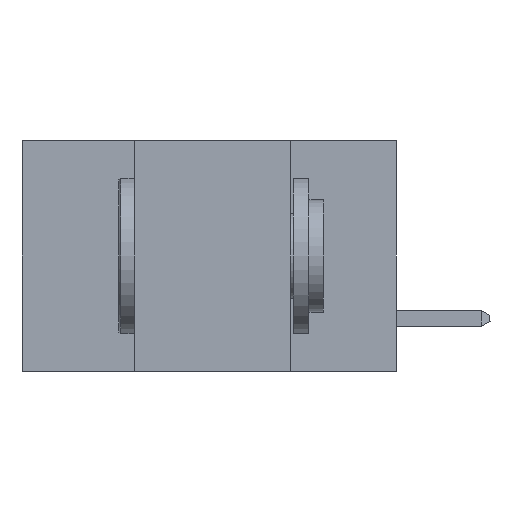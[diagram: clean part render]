
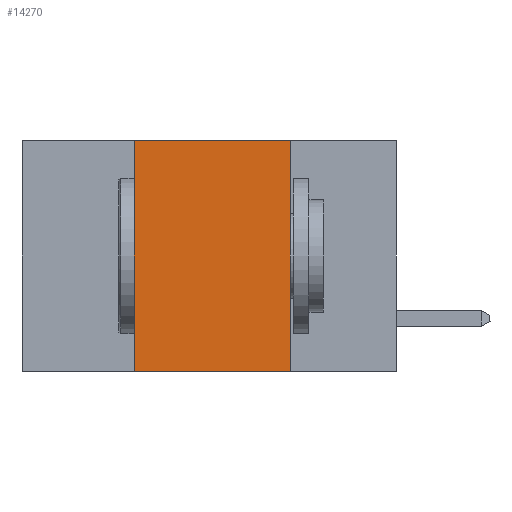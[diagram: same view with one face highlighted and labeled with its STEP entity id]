
A CAD part, left-side view. The second image highlights one B-rep face of the part: STEP entity #14270.
In plain terms, the highlighted planar face has unit normal (-1, 0, 0).
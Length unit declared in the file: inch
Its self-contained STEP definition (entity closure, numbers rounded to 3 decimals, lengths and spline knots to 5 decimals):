
#33 = DIRECTION ( 'NONE',  ( 0., 0., 1. ) ) ;
#756 = ORIENTED_EDGE ( 'NONE', *, *, #10860, .F. ) ;
#1103 = LINE ( 'NONE', #13390, #14563 ) ;
#1324 = VECTOR ( 'NONE', #15584, 39.37008 ) ;
#1913 = PLANE ( 'NONE',  #8159 ) ;
#2692 = DIRECTION ( 'NONE',  ( 0., 0., -1. ) ) ;
#3353 = DIRECTION ( 'NONE',  ( 1., 0., 0. ) ) ;
#5055 = LINE ( 'NONE', #13019, #1324 ) ;
#5102 = ORIENTED_EDGE ( 'NONE', *, *, #9111, .T. ) ;
#5184 = CARTESIAN_POINT ( 'NONE',  ( 0., 0.42, -0.37 ) ) ;
#5641 = VERTEX_POINT ( 'NONE', #5184 ) ;
#6113 = CARTESIAN_POINT ( 'NONE',  ( 0., 0.6, 0. ) ) ;
#6230 = ORIENTED_EDGE ( 'NONE', *, *, #6919, .F. ) ;
#6919 = EDGE_CURVE ( 'NONE', #15813, #9309, #8518, .T. ) ;
#8159 = AXIS2_PLACEMENT_3D ( 'NONE', #6113, #3353, #12744 ) ;
#8349 = CARTESIAN_POINT ( 'NONE',  ( 0., 0.6, 0. ) ) ;
#8485 = DIRECTION ( 'NONE',  ( 0., -1., 0. ) ) ;
#8518 = LINE ( 'NONE', #8349, #15029 ) ;
#9111 = EDGE_CURVE ( 'NONE', #5641, #13160, #5055, .T. ) ;
#9309 = VERTEX_POINT ( 'NONE', #10772 ) ;
#9647 = CARTESIAN_POINT ( 'NONE',  ( 0., 0.42, 0. ) ) ;
#10410 = FACE_OUTER_BOUND ( 'NONE', #10469, .T. ) ;
#10469 = EDGE_LOOP ( 'NONE', ( #10542, #6230, #756, #5102 ) ) ;
#10542 = ORIENTED_EDGE ( 'NONE', *, *, #12858, .F. ) ;
#10772 = CARTESIAN_POINT ( 'NONE',  ( 0., 0.17, 0. ) ) ;
#10860 = EDGE_CURVE ( 'NONE', #5641, #15813, #14699, .T. ) ;
#12744 = DIRECTION ( 'NONE',  ( 0., 0., -1. ) ) ;
#12858 = EDGE_CURVE ( 'NONE', #9309, #13160, #1103, .T. ) ;
#12930 = CARTESIAN_POINT ( 'NONE',  ( 0., 0.17, -0.37 ) ) ;
#13019 = CARTESIAN_POINT ( 'NONE',  ( 0., 0.6, -0.37 ) ) ;
#13160 = VERTEX_POINT ( 'NONE', #12930 ) ;
#13390 = CARTESIAN_POINT ( 'NONE',  ( 0., 0.17, 0. ) ) ;
#14270 = ADVANCED_FACE ( 'NONE', ( #10410 ), #1913, .F. ) ;
#14290 = VECTOR ( 'NONE', #33, 39.37008 ) ;
#14563 = VECTOR ( 'NONE', #2692, 39.37008 ) ;
#14699 = LINE ( 'NONE', #9647, #14290 ) ;
#15029 = VECTOR ( 'NONE', #8485, 39.37008 ) ;
#15584 = DIRECTION ( 'NONE',  ( 0., -1., 0. ) ) ;
#15813 = VERTEX_POINT ( 'NONE', #17032 ) ;
#17032 = CARTESIAN_POINT ( 'NONE',  ( 0., 0.42, 0. ) ) ;
